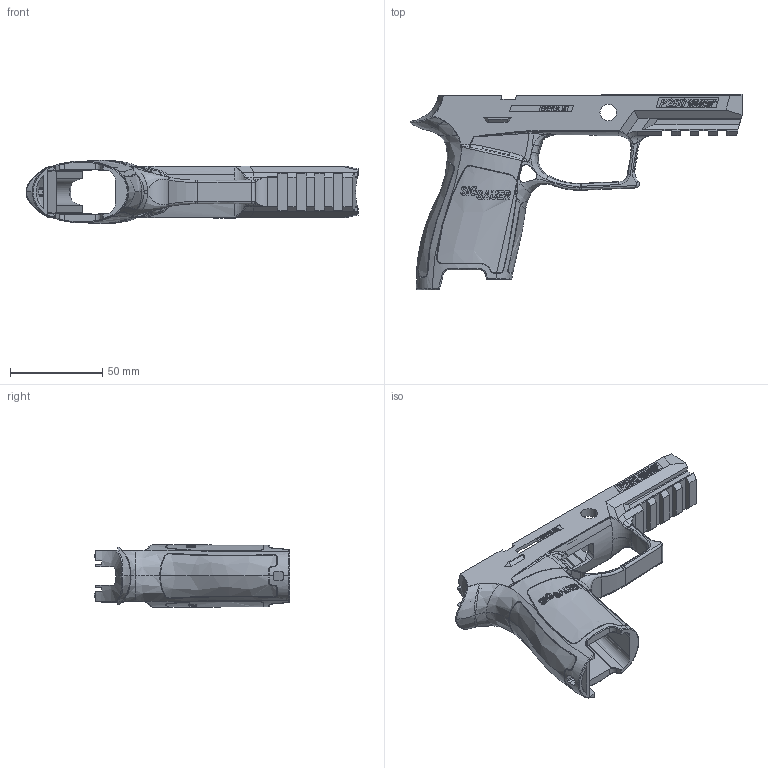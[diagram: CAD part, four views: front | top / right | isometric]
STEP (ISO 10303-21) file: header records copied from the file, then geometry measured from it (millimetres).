
FILE_DESCRIPTION (( 'STEP AP214' ), '1' );
FILE_NAME ('Polymer v5 latest backup.step', '2014-07-30T19:46:31', ( 'WarFairy' ), ( '' ), 'SwSTEP 2.0', 'SolidWorks 2013', '' );
FILE_SCHEMA (( 'AUTOMOTIVE_DESIGN' ));
Length unit declared in the file: millimetre
Products named in the file (1): Polymer v5 latest backup
Bounding box: 180.28 x 106.16 x 34.42 mm (x, y, z)
Volume: 72343.6 mm3; surface area: 45696.1 mm2
Topology: 1 solids, 1 shells, 1404 faces, 3827 edges, 2469 vertices
Faces by surface type: plane 652, bspline 603, cylinder 129, torus 18, cone 2
Entity records: 67768 total; most frequent: CARTESIAN_POINT 36990, ORIENTED_EDGE 7624, EDGE_CURVE 3812, DIRECTION 3804, VERTEX_POINT 2469, VECTOR 1898, LINE 1898, B_SPLINE_CURVE_WITH_KNOTS 1728
